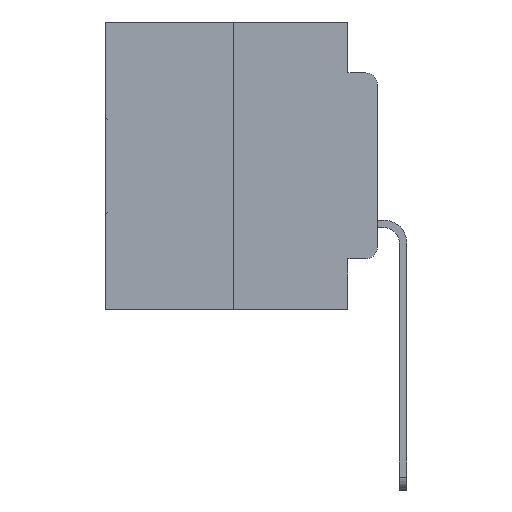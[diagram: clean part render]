
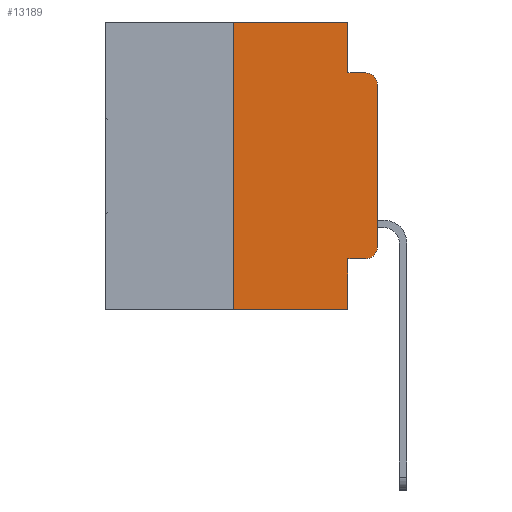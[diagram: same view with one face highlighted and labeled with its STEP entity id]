
A CAD part, left-side view. The second image highlights one B-rep face of the part: STEP entity #13189.
In plain terms, the highlighted planar face has unit normal (-1, 0, 0).
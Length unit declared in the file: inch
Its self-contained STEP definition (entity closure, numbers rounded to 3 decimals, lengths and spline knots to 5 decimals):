
#199 = ORIENTED_EDGE ( 'NONE', *, *, #4601, .T. ) ;
#405 = EDGE_CURVE ( 'NONE', #2666, #10337, #25510, .T. ) ;
#598 = VECTOR ( 'NONE', #15232, 39.37008 ) ;
#1014 = CARTESIAN_POINT ( 'NONE',  ( 0., 0., -0.1085 ) ) ;
#2105 = DIRECTION ( 'NONE',  ( -1., 0., 0. ) ) ;
#2666 = VERTEX_POINT ( 'NONE', #21714 ) ;
#4045 = DIRECTION ( 'NONE',  ( 0., -1., 0. ) ) ;
#4601 = EDGE_CURVE ( 'NONE', #23848, #5121, #24292, .T. ) ;
#4866 = CARTESIAN_POINT ( 'NONE',  ( 0., 0.473, 0. ) ) ;
#4909 = EDGE_CURVE ( 'NONE', #28223, #11866, #7679, .T. ) ;
#5121 = VERTEX_POINT ( 'NONE', #6614 ) ;
#5169 = EDGE_CURVE ( 'NONE', #28223, #2666, #16946, .T. ) ;
#5591 = CARTESIAN_POINT ( 'NONE',  ( 0., 0., -0.3915 ) ) ;
#5695 = ORIENTED_EDGE ( 'NONE', *, *, #6016, .F. ) ;
#5774 = EDGE_CURVE ( 'NONE', #10337, #11791, #30635, .T. ) ;
#5923 = EDGE_CURVE ( 'NONE', #11791, #9629, #5987, .T. ) ;
#5987 = LINE ( 'NONE', #17811, #11721 ) ;
#6016 = EDGE_CURVE ( 'NONE', #23848, #11866, #21263, .T. ) ;
#6130 = EDGE_CURVE ( 'NONE', #21017, #24916, #9827, .T. ) ;
#6230 = EDGE_CURVE ( 'NONE', #24916, #9629, #30229, .T. ) ;
#6279 = EDGE_CURVE ( 'NONE', #5121, #21017, #10206, .T. ) ;
#6614 = CARTESIAN_POINT ( 'NONE',  ( 0., 0.02, -0.4115 ) ) ;
#6659 = EDGE_LOOP ( 'NONE', ( #20187, #16926, #23154, #18431, #26017, #14785, #22450, #5695, #199, #15888 ) ) ;
#6839 = CARTESIAN_POINT ( 'NONE',  ( 0., 0.25, 0. ) ) ;
#7679 = LINE ( 'NONE', #17575, #598 ) ;
#8625 = CARTESIAN_POINT ( 'NONE',  ( 0., 0.051, 0. ) ) ;
#9288 = DIRECTION ( 'NONE',  ( 0., 0., 1. ) ) ;
#9433 = AXIS2_PLACEMENT_3D ( 'NONE', #16889, #2105, #19252 ) ;
#9629 = VERTEX_POINT ( 'NONE', #30690 ) ;
#9827 = LINE ( 'NONE', #23421, #15403 ) ;
#10206 = CIRCLE ( 'NONE', #23616, 0.02 ) ;
#10337 = VERTEX_POINT ( 'NONE', #21409 ) ;
#10695 = CARTESIAN_POINT ( 'NONE',  ( 0., 0.051, -0.5 ) ) ;
#10936 = DIRECTION ( 'NONE',  ( 1., 0., 0. ) ) ;
#11043 = DIRECTION ( 'NONE',  ( 0., 0., -1. ) ) ;
#11407 = FACE_OUTER_BOUND ( 'NONE', #6659, .T. ) ;
#11721 = VECTOR ( 'NONE', #15457, 39.37008 ) ;
#11791 = VERTEX_POINT ( 'NONE', #15247 ) ;
#11849 = VECTOR ( 'NONE', #15651, 39.37008 ) ;
#11866 = VERTEX_POINT ( 'NONE', #10695 ) ;
#12482 = CARTESIAN_POINT ( 'NONE',  ( 0., 0.02, -0.3915 ) ) ;
#13135 = VECTOR ( 'NONE', #4045, 39.37008 ) ;
#13189 = ADVANCED_FACE ( 'NONE', ( #11407 ), #24933, .F. ) ;
#14785 = ORIENTED_EDGE ( 'NONE', *, *, #5169, .F. ) ;
#14849 = DIRECTION ( 'NONE',  ( 0., 0., -1. ) ) ;
#15232 = DIRECTION ( 'NONE',  ( 0., -1., 0. ) ) ;
#15247 = CARTESIAN_POINT ( 'NONE',  ( 0., 0.051, -0.0885 ) ) ;
#15403 = VECTOR ( 'NONE', #25719, 39.37008 ) ;
#15457 = DIRECTION ( 'NONE',  ( 0., -1., 0. ) ) ;
#15651 = DIRECTION ( 'NONE',  ( 0., -1., 0. ) ) ;
#15888 = ORIENTED_EDGE ( 'NONE', *, *, #6279, .T. ) ;
#16889 = CARTESIAN_POINT ( 'NONE',  ( 0., 0.02, -0.1085 ) ) ;
#16926 = ORIENTED_EDGE ( 'NONE', *, *, #6230, .T. ) ;
#16946 = LINE ( 'NONE', #6839, #28530 ) ;
#17575 = CARTESIAN_POINT ( 'NONE',  ( 0., 0.473, -0.5 ) ) ;
#17811 = CARTESIAN_POINT ( 'NONE',  ( 0., 0.051, -0.0885 ) ) ;
#18009 = CARTESIAN_POINT ( 'NONE',  ( 0., 0.051, -0.4115 ) ) ;
#18431 = ORIENTED_EDGE ( 'NONE', *, *, #5774, .F. ) ;
#19252 = DIRECTION ( 'NONE',  ( 0., 0., -1. ) ) ;
#19637 = AXIS2_PLACEMENT_3D ( 'NONE', #20285, #10936, #27219 ) ;
#20187 = ORIENTED_EDGE ( 'NONE', *, *, #6130, .T. ) ;
#20285 = CARTESIAN_POINT ( 'NONE',  ( 0., 0.473, 0. ) ) ;
#21017 = VERTEX_POINT ( 'NONE', #5591 ) ;
#21263 = LINE ( 'NONE', #8625, #26650 ) ;
#21409 = CARTESIAN_POINT ( 'NONE',  ( 0., 0.051, 0. ) ) ;
#21714 = CARTESIAN_POINT ( 'NONE',  ( 0., 0.25, 0. ) ) ;
#22450 = ORIENTED_EDGE ( 'NONE', *, *, #4909, .T. ) ;
#23154 = ORIENTED_EDGE ( 'NONE', *, *, #5923, .F. ) ;
#23421 = CARTESIAN_POINT ( 'NONE',  ( 0., 0., 0. ) ) ;
#23616 = AXIS2_PLACEMENT_3D ( 'NONE', #12482, #28721, #14849 ) ;
#23848 = VERTEX_POINT ( 'NONE', #26517 ) ;
#24292 = LINE ( 'NONE', #18009, #11849 ) ;
#24702 = CARTESIAN_POINT ( 'NONE',  ( 0., 0.25, -0.5 ) ) ;
#24916 = VERTEX_POINT ( 'NONE', #1014 ) ;
#24933 = PLANE ( 'NONE',  #19637 ) ;
#25510 = LINE ( 'NONE', #4866, #13135 ) ;
#25719 = DIRECTION ( 'NONE',  ( 0., 0., 1. ) ) ;
#26017 = ORIENTED_EDGE ( 'NONE', *, *, #405, .F. ) ;
#26208 = CARTESIAN_POINT ( 'NONE',  ( 0., 0.051, 0. ) ) ;
#26517 = CARTESIAN_POINT ( 'NONE',  ( 0., 0.051, -0.4115 ) ) ;
#26650 = VECTOR ( 'NONE', #11043, 39.37008 ) ;
#27219 = DIRECTION ( 'NONE',  ( 0., 0., -1. ) ) ;
#28223 = VERTEX_POINT ( 'NONE', #24702 ) ;
#28530 = VECTOR ( 'NONE', #9288, 39.37008 ) ;
#28634 = DIRECTION ( 'NONE',  ( 0., 0., -1. ) ) ;
#28721 = DIRECTION ( 'NONE',  ( -1., 0., 0. ) ) ;
#29207 = VECTOR ( 'NONE', #28634, 39.37008 ) ;
#30229 = CIRCLE ( 'NONE', #9433, 0.02 ) ;
#30635 = LINE ( 'NONE', #26208, #29207 ) ;
#30690 = CARTESIAN_POINT ( 'NONE',  ( 0., 0.02, -0.0885 ) ) ;
